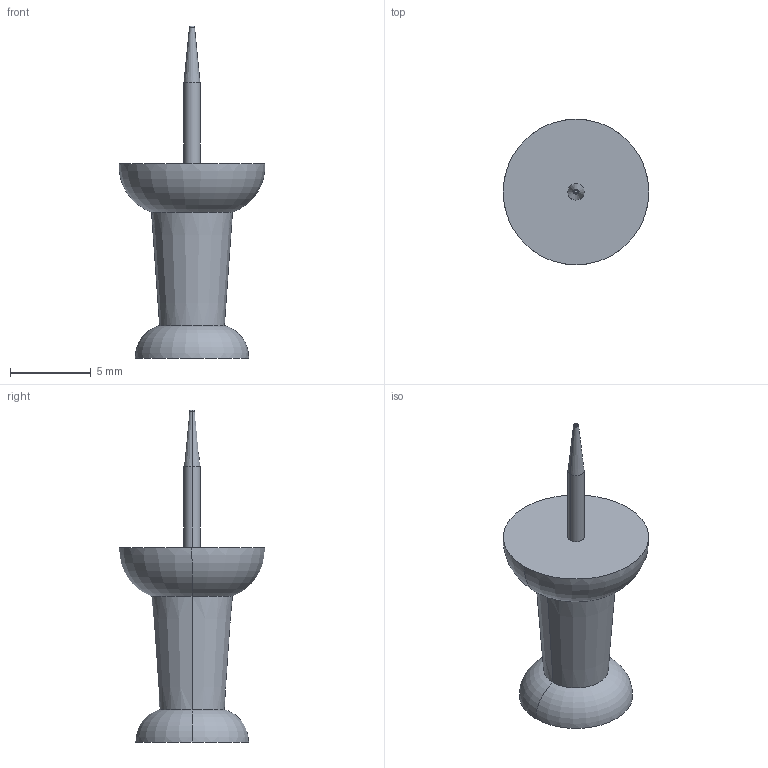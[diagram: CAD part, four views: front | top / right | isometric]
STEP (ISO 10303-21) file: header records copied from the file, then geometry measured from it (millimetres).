
FILE_DESCRIPTION (( 'STEP AP214' ), '1' );
FILE_NAME ('Thumb_Tack.STEP', '2013-11-06T14:26:53', ( 'elpi' ), ( '' ), 'SwSTEP 2.0', 'SolidWorks 2013', '' );
FILE_SCHEMA (( 'AUTOMOTIVE_DESIGN' ));
Length unit declared in the file: millimetre
Products named in the file (3): Thumb_Tack_Pin_Filed_Point; Thumb_Tack_Body; Thumb_Tack
Assembly tree (2 placements, depth 2):
  Thumb_Tack
    Thumb_Tack_Body
    Thumb_Tack_Pin_Filed_Point
Bounding box: 9 x 9 x 20.5 mm (x, y, z)
Volume: 332.3 mm3; surface area: 393.9 mm2
Topology: 2 solids, 2 shells, 19 faces, 34 edges, 20 vertices
Faces by surface type: torus 6, plane 5, cylinder 4, cone 4
Entity records: 580 total; most frequent: DIRECTION 108, CARTESIAN_POINT 78, ORIENTED_EDGE 68, AXIS2_PLACEMENT_3D 50, EDGE_CURVE 34, CIRCLE 26, VERTEX_POINT 20, EDGE_LOOP 20
